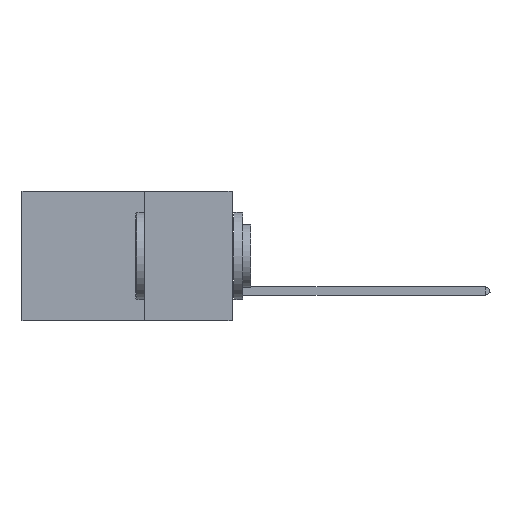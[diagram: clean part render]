
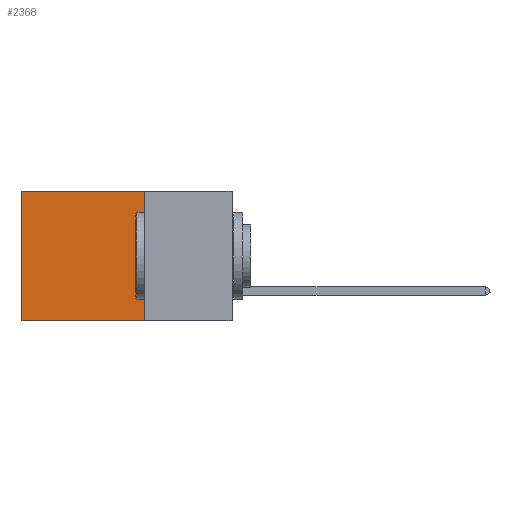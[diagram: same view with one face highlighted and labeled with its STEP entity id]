
A CAD part, left-side view. The second image highlights one B-rep face of the part: STEP entity #2368.
In plain terms, the highlighted planar face has unit normal (-1, 0, 0).
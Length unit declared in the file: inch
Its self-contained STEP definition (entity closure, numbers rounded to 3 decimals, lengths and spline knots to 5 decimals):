
#2368 = ADVANCED_FACE ( 'NONE', ( #14350 ), #28528, .F. ) ;
#2505 = EDGE_CURVE ( 'NONE', #35207, #32406, #8820, .T. ) ;
#5498 = VERTEX_POINT ( 'NONE', #12456 ) ;
#5675 = VECTOR ( 'NONE', #40168, 39.37008 ) ;
#8650 = DIRECTION ( 'NONE',  ( 0., 0., -1. ) ) ;
#8820 = LINE ( 'NONE', #13248, #41924 ) ;
#12456 = CARTESIAN_POINT ( 'NONE',  ( 0.2875, 0.6, 0. ) ) ;
#13193 = VECTOR ( 'NONE', #43318, 39.37008 ) ;
#13248 = CARTESIAN_POINT ( 'NONE',  ( 0.2875, 0.25, 0. ) ) ;
#14350 = FACE_OUTER_BOUND ( 'NONE', #43924, .T. ) ;
#15328 = CARTESIAN_POINT ( 'NONE',  ( 0.2875, 0.25, -0.37 ) ) ;
#17656 = CARTESIAN_POINT ( 'NONE',  ( 0.2875, 0.25, -0.37 ) ) ;
#18577 = LINE ( 'NONE', #44285, #5675 ) ;
#19652 = CARTESIAN_POINT ( 'NONE',  ( 0.2875, 0.25, 0. ) ) ;
#24279 = EDGE_CURVE ( 'NONE', #5498, #43198, #18577, .T. ) ;
#25669 = CARTESIAN_POINT ( 'NONE',  ( 0.2875, 0.6, -0.37 ) ) ;
#27066 = ORIENTED_EDGE ( 'NONE', *, *, #24279, .T. ) ;
#28528 = PLANE ( 'NONE',  #41349 ) ;
#29825 = DIRECTION ( 'NONE',  ( 0., 1., 0. ) ) ;
#31438 = ORIENTED_EDGE ( 'NONE', *, *, #2505, .F. ) ;
#32175 = ORIENTED_EDGE ( 'NONE', *, *, #48174, .F. ) ;
#32406 = VERTEX_POINT ( 'NONE', #15328 ) ;
#32489 = DIRECTION ( 'NONE',  ( 1., 0., 0. ) ) ;
#35207 = VERTEX_POINT ( 'NONE', #19652 ) ;
#35347 = LINE ( 'NONE', #17656, #48217 ) ;
#35964 = LINE ( 'NONE', #43148, #13193 ) ;
#39846 = CARTESIAN_POINT ( 'NONE',  ( 0.2875, 0.25, 0. ) ) ;
#40168 = DIRECTION ( 'NONE',  ( 0., 0., -1. ) ) ;
#41028 = DIRECTION ( 'NONE',  ( 0., 0., -1. ) ) ;
#41349 = AXIS2_PLACEMENT_3D ( 'NONE', #39846, #32489, #8650 ) ;
#41924 = VECTOR ( 'NONE', #41028, 39.37008 ) ;
#43148 = CARTESIAN_POINT ( 'NONE',  ( 0.2875, 0.25, 0. ) ) ;
#43198 = VERTEX_POINT ( 'NONE', #25669 ) ;
#43318 = DIRECTION ( 'NONE',  ( 0., 1., 0. ) ) ;
#43924 = EDGE_LOOP ( 'NONE', ( #27066, #32175, #31438, #47835 ) ) ;
#44285 = CARTESIAN_POINT ( 'NONE',  ( 0.2875, 0.6, 0. ) ) ;
#47835 = ORIENTED_EDGE ( 'NONE', *, *, #50239, .T. ) ;
#48174 = EDGE_CURVE ( 'NONE', #32406, #43198, #35347, .T. ) ;
#48217 = VECTOR ( 'NONE', #29825, 39.37008 ) ;
#50239 = EDGE_CURVE ( 'NONE', #35207, #5498, #35964, .T. ) ;
